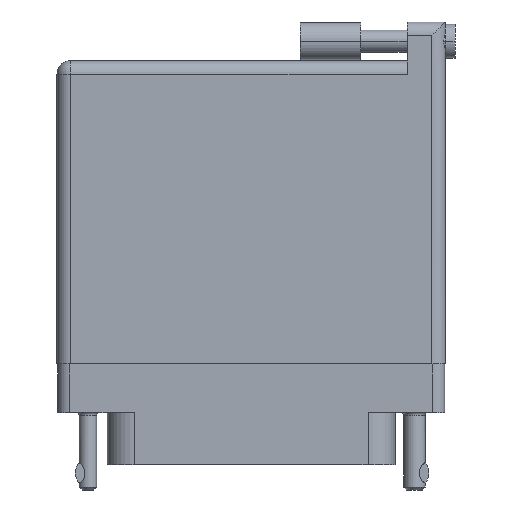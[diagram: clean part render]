
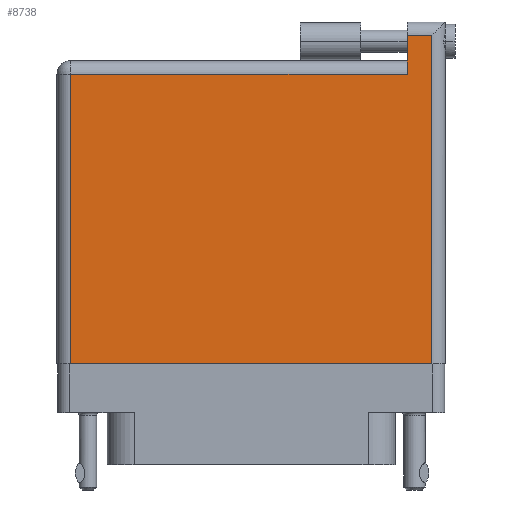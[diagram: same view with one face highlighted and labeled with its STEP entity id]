
A CAD part, front view. The second image highlights one B-rep face of the part: STEP entity #8738.
In plain terms, the highlighted face is planar.
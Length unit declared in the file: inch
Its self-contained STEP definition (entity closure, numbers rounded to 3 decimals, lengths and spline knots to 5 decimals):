
#780 = EDGE_CURVE ( 'NONE', #16560, #32178, #22571, .T. ) ;
#1308 = DIRECTION ( 'NONE',  ( 0., 1., 0. ) ) ;
#2469 = VECTOR ( 'NONE', #25364, 39.37008 ) ;
#2512 = PLANE ( 'NONE',  #19414 ) ;
#2786 = LINE ( 'NONE', #22664, #38444 ) ;
#3770 = EDGE_CURVE ( 'NONE', #33107, #16560, #32677, .T. ) ;
#3854 = FACE_OUTER_BOUND ( 'NONE', #6226, .T. ) ;
#6226 = EDGE_LOOP ( 'NONE', ( #21900, #46660, #7613, #38666, #31028, #13330 ) ) ;
#7613 = ORIENTED_EDGE ( 'NONE', *, *, #38554, .T. ) ;
#7767 = VERTEX_POINT ( 'NONE', #26367 ) ;
#8738 = ADVANCED_FACE ( 'NONE', ( #3854 ), #2512, .F. ) ;
#9293 = CARTESIAN_POINT ( 'NONE',  ( 0.934, 1.666, 0.4495 ) ) ;
#9309 = VECTOR ( 'NONE', #17549, 39.37008 ) ;
#10421 = CARTESIAN_POINT ( 'NONE',  ( -1.004, 1.396, 0.4495 ) ) ;
#10504 = DIRECTION ( 'NONE',  ( -1., 0., 0. ) ) ;
#10729 = VECTOR ( 'NONE', #41299, 39.37008 ) ;
#11348 = EDGE_CURVE ( 'NONE', #32540, #39166, #40507, .T. ) ;
#13330 = ORIENTED_EDGE ( 'NONE', *, *, #28745, .T. ) ;
#13636 = LINE ( 'NONE', #48059, #32604 ) ;
#14206 = DIRECTION ( 'NONE',  ( -1., 0., 0. ) ) ;
#16560 = VERTEX_POINT ( 'NONE', #45195 ) ;
#16626 = VECTOR ( 'NONE', #1308, 39.37008 ) ;
#17040 = LINE ( 'NONE', #36473, #9309 ) ;
#17549 = DIRECTION ( 'NONE',  ( 0., -1., 0. ) ) ;
#18295 = CARTESIAN_POINT ( 'NONE',  ( -1.004, 1.466, 0.4495 ) ) ;
#19414 = AXIS2_PLACEMENT_3D ( 'NONE', #18295, #44881, #10504 ) ;
#19982 = CARTESIAN_POINT ( 'NONE',  ( 0.934, 1.596, 0.4495 ) ) ;
#21900 = ORIENTED_EDGE ( 'NONE', *, *, #3770, .T. ) ;
#22571 = LINE ( 'NONE', #9293, #16626 ) ;
#22664 = CARTESIAN_POINT ( 'NONE',  ( -0.934, -0.1, 0.4495 ) ) ;
#25364 = DIRECTION ( 'NONE',  ( -1., 0., 0. ) ) ;
#26206 = CARTESIAN_POINT ( 'NONE',  ( -1.004, -0.1, 0.4495 ) ) ;
#26367 = CARTESIAN_POINT ( 'NONE',  ( 0.807, 1.596, 0.4495 ) ) ;
#28745 = EDGE_CURVE ( 'NONE', #39166, #33107, #2786, .T. ) ;
#28935 = CARTESIAN_POINT ( 'NONE',  ( 0.807, 1.396, 0.4495 ) ) ;
#31028 = ORIENTED_EDGE ( 'NONE', *, *, #11348, .T. ) ;
#31532 = CARTESIAN_POINT ( 'NONE',  ( -0.934, 1.396, 0.4495 ) ) ;
#32178 = VERTEX_POINT ( 'NONE', #19982 ) ;
#32540 = VERTEX_POINT ( 'NONE', #28935 ) ;
#32604 = VECTOR ( 'NONE', #14206, 39.37008 ) ;
#32677 = LINE ( 'NONE', #26206, #10729 ) ;
#33107 = VERTEX_POINT ( 'NONE', #44485 ) ;
#36473 = CARTESIAN_POINT ( 'NONE',  ( 0.807, 1.666, 0.4495 ) ) ;
#38444 = VECTOR ( 'NONE', #41752, 39.37008 ) ;
#38554 = EDGE_CURVE ( 'NONE', #32178, #7767, #13636, .T. ) ;
#38666 = ORIENTED_EDGE ( 'NONE', *, *, #41544, .T. ) ;
#39166 = VERTEX_POINT ( 'NONE', #31532 ) ;
#40507 = LINE ( 'NONE', #10421, #2469 ) ;
#41299 = DIRECTION ( 'NONE',  ( 1., 0., 0. ) ) ;
#41544 = EDGE_CURVE ( 'NONE', #7767, #32540, #17040, .T. ) ;
#41752 = DIRECTION ( 'NONE',  ( 0., -1., 0. ) ) ;
#44485 = CARTESIAN_POINT ( 'NONE',  ( -0.934, -0.1, 0.4495 ) ) ;
#44881 = DIRECTION ( 'NONE',  ( 0., 0., -1. ) ) ;
#45195 = CARTESIAN_POINT ( 'NONE',  ( 0.934, -0.1, 0.4495 ) ) ;
#46660 = ORIENTED_EDGE ( 'NONE', *, *, #780, .T. ) ;
#48059 = CARTESIAN_POINT ( 'NONE',  ( -1.004, 1.596, 0.4495 ) ) ;
